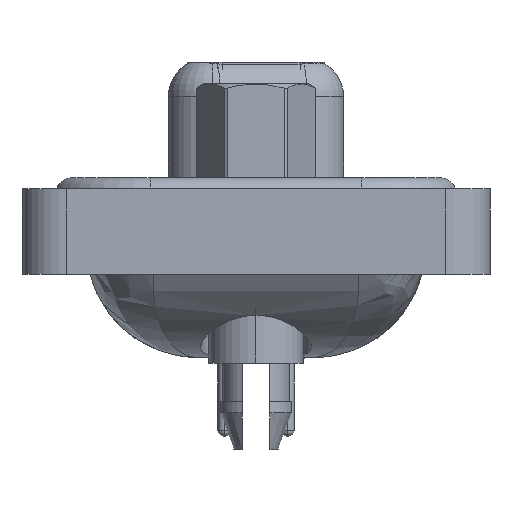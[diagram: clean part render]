
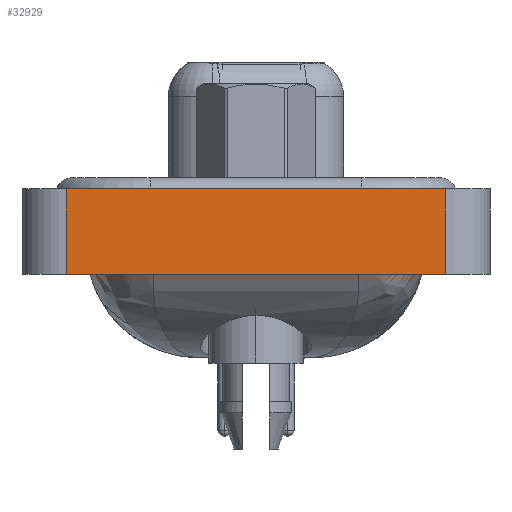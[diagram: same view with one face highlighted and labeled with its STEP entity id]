
A CAD part, left-side view. The second image highlights one B-rep face of the part: STEP entity #32929.
In plain terms, the highlighted planar face has unit normal (-1, 0, 0).
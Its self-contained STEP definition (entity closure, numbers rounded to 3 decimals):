
#198 = VECTOR ( 'NONE', #24947, 1000. ) ;
#2972 = EDGE_LOOP ( 'NONE', ( #8255, #26389, #3610, #20622 ) ) ;
#3211 = CARTESIAN_POINT ( 'NONE',  ( -7.15, -8.55, 0.5 ) ) ;
#3359 = FACE_OUTER_BOUND ( 'NONE', #2972, .T. ) ;
#3413 = CARTESIAN_POINT ( 'NONE',  ( -7.15, 8.55, 0.5 ) ) ;
#3571 = VECTOR ( 'NONE', #21863, 1000. ) ;
#3610 = ORIENTED_EDGE ( 'NONE', *, *, #23504, .F. ) ;
#4089 = CARTESIAN_POINT ( 'NONE',  ( -7.15, 8.55, -3.35 ) ) ;
#5427 = CARTESIAN_POINT ( 'NONE',  ( -7.15, 8.55, -3.35 ) ) ;
#5811 = CARTESIAN_POINT ( 'NONE',  ( -7.15, -8.55, -3.35 ) ) ;
#7482 = EDGE_CURVE ( 'NONE', #21545, #10105, #30332, .T. ) ;
#7675 = VERTEX_POINT ( 'NONE', #4089 ) ;
#8255 = ORIENTED_EDGE ( 'NONE', *, *, #7482, .T. ) ;
#10105 = VERTEX_POINT ( 'NONE', #3211 ) ;
#13460 = DIRECTION ( 'NONE',  ( 0., 0., 1. ) ) ;
#13667 = LINE ( 'NONE', #5811, #3571 ) ;
#14406 = DIRECTION ( 'NONE',  ( 0., 0., 1. ) ) ;
#16594 = CARTESIAN_POINT ( 'NONE',  ( -7.15, -8.55, -3.35 ) ) ;
#19766 = DIRECTION ( 'NONE',  ( -1., 0., 0. ) ) ;
#20274 = CARTESIAN_POINT ( 'NONE',  ( -7.15, -8.55, -3.35 ) ) ;
#20622 = ORIENTED_EDGE ( 'NONE', *, *, #26948, .T. ) ;
#21545 = VERTEX_POINT ( 'NONE', #20274 ) ;
#21863 = DIRECTION ( 'NONE',  ( 0., -1., 0. ) ) ;
#23504 = EDGE_CURVE ( 'NONE', #7675, #30110, #24148, .T. ) ;
#24148 = LINE ( 'NONE', #5427, #24524 ) ;
#24524 = VECTOR ( 'NONE', #13460, 1000. ) ;
#24947 = DIRECTION ( 'NONE',  ( 0., 0., 1. ) ) ;
#25099 = PLANE ( 'NONE',  #32952 ) ;
#26178 = DIRECTION ( 'NONE',  ( 0., -1., 0. ) ) ;
#26389 = ORIENTED_EDGE ( 'NONE', *, *, #32968, .F. ) ;
#26948 = EDGE_CURVE ( 'NONE', #7675, #21545, #13667, .T. ) ;
#30110 = VERTEX_POINT ( 'NONE', #3413 ) ;
#30138 = CARTESIAN_POINT ( 'NONE',  ( -7.15, -8.55, -3.35 ) ) ;
#30332 = LINE ( 'NONE', #16594, #198 ) ;
#31203 = LINE ( 'NONE', #31555, #34098 ) ;
#31555 = CARTESIAN_POINT ( 'NONE',  ( -7.15, -8.55, 0.5 ) ) ;
#32929 = ADVANCED_FACE ( 'NONE', ( #3359 ), #25099, .T. ) ;
#32952 = AXIS2_PLACEMENT_3D ( 'NONE', #30138, #19766, #14406 ) ;
#32968 = EDGE_CURVE ( 'NONE', #30110, #10105, #31203, .T. ) ;
#34098 = VECTOR ( 'NONE', #26178, 1000. ) ;
